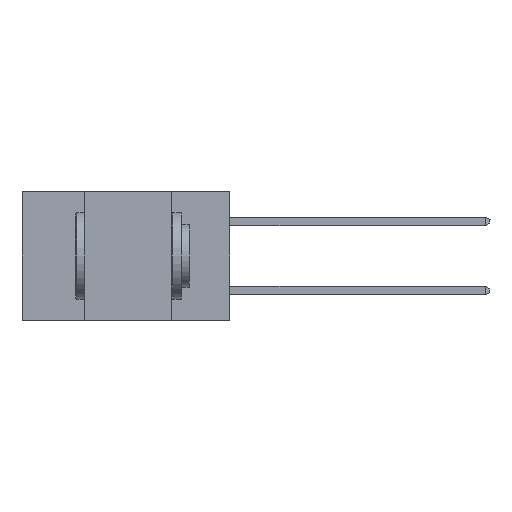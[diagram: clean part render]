
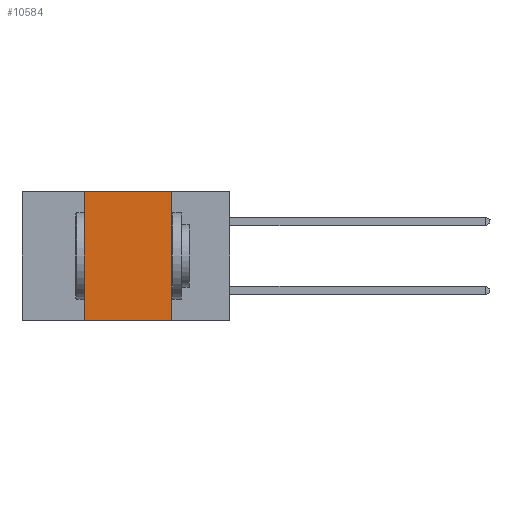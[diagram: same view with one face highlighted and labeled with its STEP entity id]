
A CAD part, left-side view. The second image highlights one B-rep face of the part: STEP entity #10584.
In plain terms, the highlighted planar face has unit normal (-1, 0, 0).
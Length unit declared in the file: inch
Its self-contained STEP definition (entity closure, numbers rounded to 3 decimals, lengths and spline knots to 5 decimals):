
#619 = DIRECTION ( 'NONE',  ( 0., 0., -1. ) ) ;
#862 = CARTESIAN_POINT ( 'NONE',  ( 0., 0.17, -0.37 ) ) ;
#1335 = LINE ( 'NONE', #862, #19973 ) ;
#1408 = CARTESIAN_POINT ( 'NONE',  ( 0., 0.6, -0.37 ) ) ;
#1681 = VECTOR ( 'NONE', #18596, 39.37008 ) ;
#2035 = EDGE_LOOP ( 'NONE', ( #20073, #14619, #16912, #13123 ) ) ;
#4459 = VERTEX_POINT ( 'NONE', #17245 ) ;
#4792 = VERTEX_POINT ( 'NONE', #20411 ) ;
#4994 = DIRECTION ( 'NONE',  ( 0., -1., 0. ) ) ;
#6150 = EDGE_CURVE ( 'NONE', #10088, #4792, #10725, .T. ) ;
#6778 = LINE ( 'NONE', #1408, #12205 ) ;
#7685 = DIRECTION ( 'NONE',  ( 0., -1., 0. ) ) ;
#8532 = AXIS2_PLACEMENT_3D ( 'NONE', #20874, #10178, #619 ) ;
#10088 = VERTEX_POINT ( 'NONE', #13113 ) ;
#10178 = DIRECTION ( 'NONE',  ( 1., 0., 0. ) ) ;
#10584 = ADVANCED_FACE ( 'NONE', ( #15437 ), #13633, .F. ) ;
#10725 = LINE ( 'NONE', #13181, #22904 ) ;
#10860 = EDGE_CURVE ( 'NONE', #22282, #10088, #21938, .T. ) ;
#12205 = VECTOR ( 'NONE', #4994, 39.37008 ) ;
#12906 = CARTESIAN_POINT ( 'NONE',  ( 0., 0.42, -0.37 ) ) ;
#13113 = CARTESIAN_POINT ( 'NONE',  ( 0., 0.42, 0. ) ) ;
#13123 = ORIENTED_EDGE ( 'NONE', *, *, #23185, .T. ) ;
#13181 = CARTESIAN_POINT ( 'NONE',  ( 0., 0.6, 0. ) ) ;
#13633 = PLANE ( 'NONE',  #8532 ) ;
#13784 = EDGE_CURVE ( 'NONE', #4792, #4459, #1335, .T. ) ;
#14619 = ORIENTED_EDGE ( 'NONE', *, *, #6150, .F. ) ;
#15437 = FACE_OUTER_BOUND ( 'NONE', #2035, .T. ) ;
#16912 = ORIENTED_EDGE ( 'NONE', *, *, #10860, .F. ) ;
#17123 = CARTESIAN_POINT ( 'NONE',  ( 0., 0.42, -0.37 ) ) ;
#17245 = CARTESIAN_POINT ( 'NONE',  ( 0., 0.17, -0.37 ) ) ;
#18596 = DIRECTION ( 'NONE',  ( 0., 0., 1. ) ) ;
#19973 = VECTOR ( 'NONE', #20759, 39.37008 ) ;
#20073 = ORIENTED_EDGE ( 'NONE', *, *, #13784, .F. ) ;
#20411 = CARTESIAN_POINT ( 'NONE',  ( 0., 0.17, 0. ) ) ;
#20759 = DIRECTION ( 'NONE',  ( 0., 0., -1. ) ) ;
#20874 = CARTESIAN_POINT ( 'NONE',  ( 0., 0.6, 0. ) ) ;
#21938 = LINE ( 'NONE', #12906, #1681 ) ;
#22282 = VERTEX_POINT ( 'NONE', #17123 ) ;
#22904 = VECTOR ( 'NONE', #7685, 39.37008 ) ;
#23185 = EDGE_CURVE ( 'NONE', #22282, #4459, #6778, .T. ) ;
